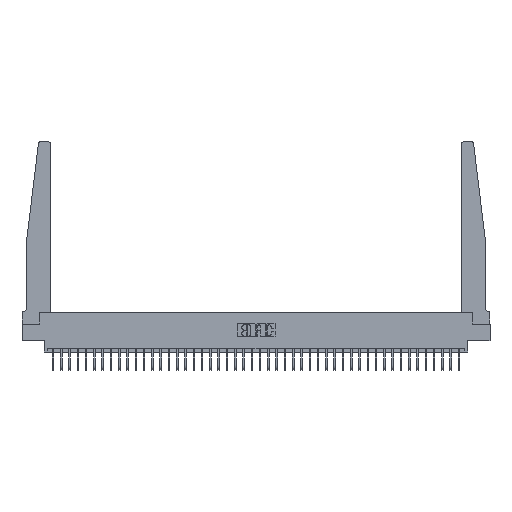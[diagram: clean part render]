
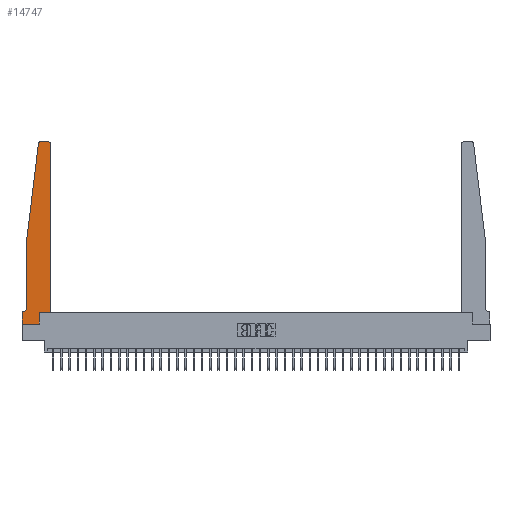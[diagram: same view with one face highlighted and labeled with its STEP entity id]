
A CAD part, top view. The second image highlights one B-rep face of the part: STEP entity #14747.
In plain terms, the highlighted planar face has unit normal (0, 0, 1).
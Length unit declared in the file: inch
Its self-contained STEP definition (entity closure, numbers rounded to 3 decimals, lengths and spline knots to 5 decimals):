
#153 = ORIENTED_EDGE ( 'NONE', *, *, #17939, .T. ) ;
#518 = VERTEX_POINT ( 'NONE', #3713 ) ;
#542 = VECTOR ( 'NONE', #7469, 39.37008 ) ;
#671 = DIRECTION ( 'NONE',  ( 0., -1., 0. ) ) ;
#1081 = EDGE_CURVE ( 'NONE', #7273, #2750, #26259, .T. ) ;
#1341 = CARTESIAN_POINT ( 'NONE',  ( 0.425, 2.72, 0.37 ) ) ;
#1507 = EDGE_CURVE ( 'NONE', #6084, #6583, #30341, .T. ) ;
#2339 = CIRCLE ( 'NONE', #21798, 0.05 ) ;
#2750 = VERTEX_POINT ( 'NONE', #10035 ) ;
#3713 = CARTESIAN_POINT ( 'NONE',  ( 0.395, 2.75, 0.37 ) ) ;
#3832 = CARTESIAN_POINT ( 'NONE',  ( 0.27653, 2.72, 0.37 ) ) ;
#4490 = DIRECTION ( 'NONE',  ( 0., 1., 0. ) ) ;
#4938 = CARTESIAN_POINT ( 'NONE',  ( 0.2605, 0., 0.37 ) ) ;
#5774 = VERTEX_POINT ( 'NONE', #24066 ) ;
#5794 = AXIS2_PLACEMENT_3D ( 'NONE', #29924, #35602, #26591 ) ;
#6084 = VERTEX_POINT ( 'NONE', #8773 ) ;
#6439 = ORIENTED_EDGE ( 'NONE', *, *, #10431, .T. ) ;
#6583 = VERTEX_POINT ( 'NONE', #33541 ) ;
#6668 = VERTEX_POINT ( 'NONE', #14916 ) ;
#7244 = AXIS2_PLACEMENT_3D ( 'NONE', #35628, #15044, #20903 ) ;
#7273 = VERTEX_POINT ( 'NONE', #4938 ) ;
#7469 = DIRECTION ( 'NONE',  ( -1., 0., 0. ) ) ;
#7758 = ORIENTED_EDGE ( 'NONE', *, *, #22468, .T. ) ;
#7944 = LINE ( 'NONE', #13292, #542 ) ;
#8128 = LINE ( 'NONE', #36261, #22533 ) ;
#8312 = VERTEX_POINT ( 'NONE', #9777 ) ;
#8773 = CARTESIAN_POINT ( 'NONE',  ( 0.015, 0.1875, 0.37 ) ) ;
#8908 = LINE ( 'NONE', #13380, #24690 ) ;
#8943 = CARTESIAN_POINT ( 'NONE',  ( 0.065, 1.25, 0.37 ) ) ;
#9242 = LINE ( 'NONE', #8943, #31960 ) ;
#9418 = DIRECTION ( 'NONE',  ( -1., 0., 0. ) ) ;
#9584 = DIRECTION ( 'NONE',  ( 0., -1., 0. ) ) ;
#9777 = CARTESIAN_POINT ( 'NONE',  ( 0.065, 1.25, 0.37 ) ) ;
#10035 = CARTESIAN_POINT ( 'NONE',  ( 0.2605, 0.18, 0.37 ) ) ;
#10431 = EDGE_CURVE ( 'NONE', #6668, #12050, #16044, .T. ) ;
#12050 = VERTEX_POINT ( 'NONE', #1341 ) ;
#12224 = DIRECTION ( 'NONE',  ( 0., 0., 1. ) ) ;
#13048 = VERTEX_POINT ( 'NONE', #14705 ) ;
#13169 = DIRECTION ( 'NONE',  ( 0., 1., 0. ) ) ;
#13292 = CARTESIAN_POINT ( 'NONE',  ( 0.25, 2.75, 0.37 ) ) ;
#13380 = CARTESIAN_POINT ( 'NONE',  ( 0., 0., 0.37 ) ) ;
#13864 = EDGE_LOOP ( 'NONE', ( #153, #37962, #22600, #7758, #25878, #23951, #29123, #35740, #26261, #29295, #6439, #24890 ) ) ;
#14649 = PLANE ( 'NONE',  #5794 ) ;
#14705 = CARTESIAN_POINT ( 'NONE',  ( 0.27653, 2.75, 0.37 ) ) ;
#14747 = ADVANCED_FACE ( 'NONE', ( #28294 ), #14649, .T. ) ;
#14916 = CARTESIAN_POINT ( 'NONE',  ( 0.425, 0.18, 0.37 ) ) ;
#15044 = DIRECTION ( 'NONE',  ( 0., 0., 1. ) ) ;
#16044 = LINE ( 'NONE', #31704, #23027 ) ;
#16333 = DIRECTION ( 'NONE',  ( 1., 0., 0. ) ) ;
#16914 = VECTOR ( 'NONE', #26783, 39.37008 ) ;
#17302 = CARTESIAN_POINT ( 'NONE',  ( 0.425, 0.18, 0.37 ) ) ;
#17939 = EDGE_CURVE ( 'NONE', #518, #13048, #7944, .T. ) ;
#18253 = EDGE_CURVE ( 'NONE', #13048, #5774, #23686, .T. ) ;
#18511 = DIRECTION ( 'NONE',  ( -0.122, -0.992, 0. ) ) ;
#19031 = EDGE_CURVE ( 'NONE', #21893, #6084, #2339, .T. ) ;
#20541 = CIRCLE ( 'NONE', #7244, 0.03 ) ;
#20675 = VECTOR ( 'NONE', #4490, 39.37008 ) ;
#20903 = DIRECTION ( 'NONE',  ( 1., 0., 0. ) ) ;
#21256 = DIRECTION ( 'NONE',  ( 0., 0., -1. ) ) ;
#21377 = VECTOR ( 'NONE', #26160, 39.37008 ) ;
#21673 = EDGE_CURVE ( 'NONE', #6583, #24046, #8128, .T. ) ;
#21676 = CARTESIAN_POINT ( 'NONE',  ( 0.065, 0.2375, 0.37 ) ) ;
#21798 = AXIS2_PLACEMENT_3D ( 'NONE', #24741, #21256, #9418 ) ;
#21893 = VERTEX_POINT ( 'NONE', #21676 ) ;
#21977 = LINE ( 'NONE', #36349, #23838 ) ;
#22468 = EDGE_CURVE ( 'NONE', #8312, #21893, #21977, .T. ) ;
#22533 = VECTOR ( 'NONE', #9584, 39.37008 ) ;
#22600 = ORIENTED_EDGE ( 'NONE', *, *, #28685, .T. ) ;
#23027 = VECTOR ( 'NONE', #13169, 39.37008 ) ;
#23686 = CIRCLE ( 'NONE', #35366, 0.03 ) ;
#23838 = VECTOR ( 'NONE', #671, 39.37008 ) ;
#23951 = ORIENTED_EDGE ( 'NONE', *, *, #1507, .T. ) ;
#24046 = VERTEX_POINT ( 'NONE', #31715 ) ;
#24066 = CARTESIAN_POINT ( 'NONE',  ( 0.24675, 2.72367, 0.37 ) ) ;
#24690 = VECTOR ( 'NONE', #16333, 39.37008 ) ;
#24741 = CARTESIAN_POINT ( 'NONE',  ( 0.015, 0.2375, 0.37 ) ) ;
#24890 = ORIENTED_EDGE ( 'NONE', *, *, #36440, .T. ) ;
#25878 = ORIENTED_EDGE ( 'NONE', *, *, #19031, .T. ) ;
#26160 = DIRECTION ( 'NONE',  ( 1., 0., 0. ) ) ;
#26259 = LINE ( 'NONE', #30980, #20675 ) ;
#26261 = ORIENTED_EDGE ( 'NONE', *, *, #1081, .T. ) ;
#26591 = DIRECTION ( 'NONE',  ( 1., 0., 0. ) ) ;
#26783 = DIRECTION ( 'NONE',  ( -1., 0., 0. ) ) ;
#27249 = CARTESIAN_POINT ( 'NONE',  ( 0.065, 0.1875, 0.37 ) ) ;
#27388 = DIRECTION ( 'NONE',  ( 1., 0., 0. ) ) ;
#28294 = FACE_OUTER_BOUND ( 'NONE', #13864, .T. ) ;
#28685 = EDGE_CURVE ( 'NONE', #5774, #8312, #9242, .T. ) ;
#29123 = ORIENTED_EDGE ( 'NONE', *, *, #21673, .T. ) ;
#29295 = ORIENTED_EDGE ( 'NONE', *, *, #31755, .T. ) ;
#29924 = CARTESIAN_POINT ( 'NONE',  ( 0., 0.1875, 0.37 ) ) ;
#30341 = LINE ( 'NONE', #27249, #16914 ) ;
#30980 = CARTESIAN_POINT ( 'NONE',  ( 0.2605, 0.18, 0.37 ) ) ;
#31704 = CARTESIAN_POINT ( 'NONE',  ( 0.425, 0.18, 0.37 ) ) ;
#31715 = CARTESIAN_POINT ( 'NONE',  ( 0., 0., 0.37 ) ) ;
#31755 = EDGE_CURVE ( 'NONE', #2750, #6668, #34320, .T. ) ;
#31960 = VECTOR ( 'NONE', #18511, 39.37008 ) ;
#33541 = CARTESIAN_POINT ( 'NONE',  ( 0., 0.1875, 0.37 ) ) ;
#34320 = LINE ( 'NONE', #17302, #21377 ) ;
#35366 = AXIS2_PLACEMENT_3D ( 'NONE', #3832, #12224, #27388 ) ;
#35602 = DIRECTION ( 'NONE',  ( 0., 0., 1. ) ) ;
#35628 = CARTESIAN_POINT ( 'NONE',  ( 0.395, 2.72, 0.37 ) ) ;
#35740 = ORIENTED_EDGE ( 'NONE', *, *, #36572, .T. ) ;
#36261 = CARTESIAN_POINT ( 'NONE',  ( 0., 0., 0.37 ) ) ;
#36349 = CARTESIAN_POINT ( 'NONE',  ( 0.065, 1.25, 0.37 ) ) ;
#36440 = EDGE_CURVE ( 'NONE', #12050, #518, #20541, .T. ) ;
#36572 = EDGE_CURVE ( 'NONE', #24046, #7273, #8908, .T. ) ;
#37962 = ORIENTED_EDGE ( 'NONE', *, *, #18253, .T. ) ;
